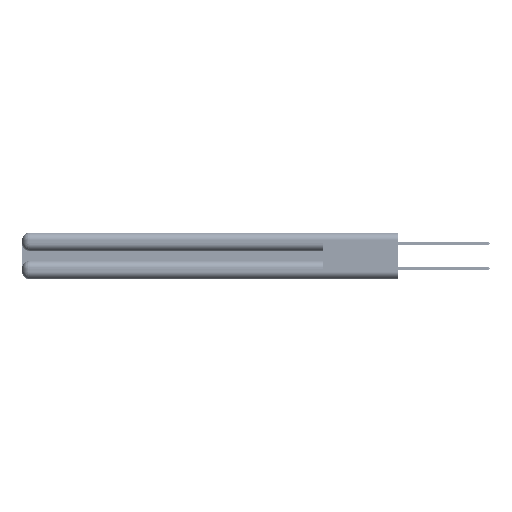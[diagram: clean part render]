
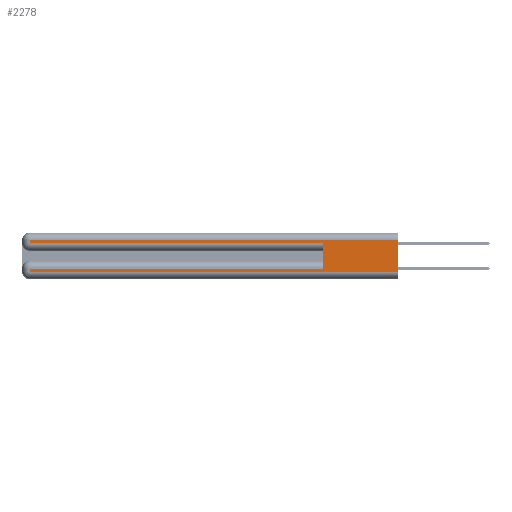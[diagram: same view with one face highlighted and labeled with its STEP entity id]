
A CAD part, left-side view. The second image highlights one B-rep face of the part: STEP entity #2278.
In plain terms, the highlighted planar face has unit normal (-1, 0, 0).
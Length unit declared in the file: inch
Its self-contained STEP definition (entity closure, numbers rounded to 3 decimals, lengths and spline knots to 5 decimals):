
#260 = VECTOR ( 'NONE', #47525, 39.37008 ) ;
#1734 = DIRECTION ( 'NONE',  ( 1., 0., 0. ) ) ;
#2278 = ADVANCED_FACE ( 'NONE', ( #47710 ), #50868, .F. ) ;
#2493 = CARTESIAN_POINT ( 'NONE',  ( 0., 0., 0.06 ) ) ;
#3386 = EDGE_LOOP ( 'NONE', ( #31779, #14804, #8898, #6642, #47773, #31325, #37272, #37436 ) ) ;
#4611 = EDGE_CURVE ( 'NONE', #15177, #32440, #8957, .T. ) ;
#4801 = CARTESIAN_POINT ( 'NONE',  ( 0., 0., 0.285 ) ) ;
#5191 = CARTESIAN_POINT ( 'NONE',  ( 0., 2.94, 0.31 ) ) ;
#5335 = EDGE_CURVE ( 'NONE', #22215, #37289, #29957, .T. ) ;
#6642 = ORIENTED_EDGE ( 'NONE', *, *, #4611, .T. ) ;
#6750 = CARTESIAN_POINT ( 'NONE',  ( 0., 0., 0.06 ) ) ;
#8898 = ORIENTED_EDGE ( 'NONE', *, *, #44362, .T. ) ;
#8943 = DIRECTION ( 'NONE',  ( 0., -1., 0. ) ) ;
#8957 = LINE ( 'NONE', #4801, #30692 ) ;
#9401 = VECTOR ( 'NONE', #32811, 39.37008 ) ;
#10195 = LINE ( 'NONE', #21615, #30654 ) ;
#12221 = VECTOR ( 'NONE', #42384, 39.37008 ) ;
#14804 = ORIENTED_EDGE ( 'NONE', *, *, #28067, .T. ) ;
#15177 = VERTEX_POINT ( 'NONE', #25958 ) ;
#16082 = EDGE_CURVE ( 'NONE', #37289, #30857, #32000, .T. ) ;
#16108 = CARTESIAN_POINT ( 'NONE',  ( 0., 2.94, 0.085 ) ) ;
#16849 = VERTEX_POINT ( 'NONE', #35964 ) ;
#17079 = DIRECTION ( 'NONE',  ( 0., 0., -1. ) ) ;
#17808 = VECTOR ( 'NONE', #17079, 39.37008 ) ;
#18807 = EDGE_CURVE ( 'NONE', #16849, #32440, #40065, .T. ) ;
#21136 = VERTEX_POINT ( 'NONE', #5191 ) ;
#21170 = CARTESIAN_POINT ( 'NONE',  ( 0., 2.94, 0.37 ) ) ;
#21615 = CARTESIAN_POINT ( 'NONE',  ( 0., 0., 0.31 ) ) ;
#22142 = CARTESIAN_POINT ( 'NONE',  ( 0., 0., 0.37 ) ) ;
#22215 = VERTEX_POINT ( 'NONE', #16108 ) ;
#24429 = CARTESIAN_POINT ( 'NONE',  ( 0., 0.6, 0.145 ) ) ;
#25751 = DIRECTION ( 'NONE',  ( 0., 1., 0. ) ) ;
#25841 = CARTESIAN_POINT ( 'NONE',  ( 0., 0., 0.37 ) ) ;
#25958 = CARTESIAN_POINT ( 'NONE',  ( 0., 2.94, 0.285 ) ) ;
#26224 = VERTEX_POINT ( 'NONE', #26299 ) ;
#26299 = CARTESIAN_POINT ( 'NONE',  ( 0., 0., 0.31 ) ) ;
#27036 = DIRECTION ( 'NONE',  ( 0., -1., 0. ) ) ;
#28067 = EDGE_CURVE ( 'NONE', #26224, #21136, #10195, .T. ) ;
#28654 = CARTESIAN_POINT ( 'NONE',  ( 0., 0., 0.085 ) ) ;
#29957 = LINE ( 'NONE', #21170, #17808 ) ;
#30393 = DIRECTION ( 'NONE',  ( 0., 0., -1. ) ) ;
#30654 = VECTOR ( 'NONE', #25751, 39.37008 ) ;
#30692 = VECTOR ( 'NONE', #8943, 39.37008 ) ;
#30857 = VERTEX_POINT ( 'NONE', #6750 ) ;
#31325 = ORIENTED_EDGE ( 'NONE', *, *, #36801, .T. ) ;
#31501 = CARTESIAN_POINT ( 'NONE',  ( 0., 2.94, 0.06 ) ) ;
#31779 = ORIENTED_EDGE ( 'NONE', *, *, #51331, .F. ) ;
#32000 = LINE ( 'NONE', #2493, #41633 ) ;
#32440 = VERTEX_POINT ( 'NONE', #48481 ) ;
#32455 = LINE ( 'NONE', #28654, #9401 ) ;
#32811 = DIRECTION ( 'NONE',  ( 0., 1., 0. ) ) ;
#33389 = VECTOR ( 'NONE', #35714, 39.37008 ) ;
#35714 = DIRECTION ( 'NONE',  ( 0., 0., -1. ) ) ;
#35964 = CARTESIAN_POINT ( 'NONE',  ( 0., 0.6, 0.085 ) ) ;
#36801 = EDGE_CURVE ( 'NONE', #16849, #22215, #32455, .T. ) ;
#37272 = ORIENTED_EDGE ( 'NONE', *, *, #5335, .T. ) ;
#37289 = VERTEX_POINT ( 'NONE', #31501 ) ;
#37436 = ORIENTED_EDGE ( 'NONE', *, *, #16082, .T. ) ;
#40065 = LINE ( 'NONE', #24429, #260 ) ;
#41633 = VECTOR ( 'NONE', #27036, 39.37008 ) ;
#42384 = DIRECTION ( 'NONE',  ( 0., 0., -1. ) ) ;
#43793 = CARTESIAN_POINT ( 'NONE',  ( 0., 2.94, 0.37 ) ) ;
#44324 = LINE ( 'NONE', #43793, #33389 ) ;
#44362 = EDGE_CURVE ( 'NONE', #21136, #15177, #44324, .T. ) ;
#44909 = LINE ( 'NONE', #25841, #12221 ) ;
#45735 = AXIS2_PLACEMENT_3D ( 'NONE', #22142, #1734, #30393 ) ;
#47525 = DIRECTION ( 'NONE',  ( 0., 0., 1. ) ) ;
#47710 = FACE_OUTER_BOUND ( 'NONE', #3386, .T. ) ;
#47773 = ORIENTED_EDGE ( 'NONE', *, *, #18807, .F. ) ;
#48481 = CARTESIAN_POINT ( 'NONE',  ( 0., 0.6, 0.285 ) ) ;
#50868 = PLANE ( 'NONE',  #45735 ) ;
#51331 = EDGE_CURVE ( 'NONE', #26224, #30857, #44909, .T. ) ;
